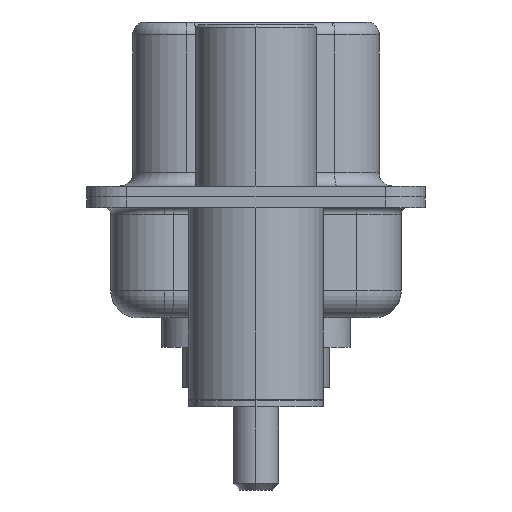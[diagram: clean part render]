
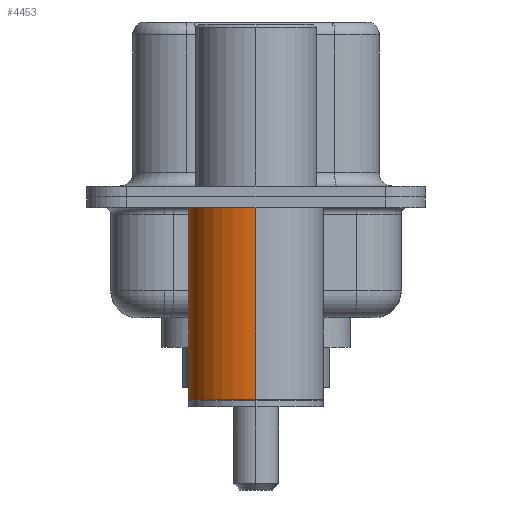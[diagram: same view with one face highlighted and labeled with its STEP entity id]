
A CAD part, left-side view. The second image highlights one B-rep face of the part: STEP entity #4453.
In plain terms, the highlighted cylindrical face has radius 2.5 mm (diameter 5 mm), a partial arc.
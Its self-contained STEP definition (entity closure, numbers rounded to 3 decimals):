
#446 = ORIENTED_EDGE ( 'NONE', *, *, #5143, .F. ) ;
#450 = CARTESIAN_POINT ( 'NONE',  ( 0., 0., -7.525 ) ) ;
#824 = VERTEX_POINT ( 'NONE', #5854 ) ;
#1178 = EDGE_LOOP ( 'NONE', ( #3720, #10890, #16262, #446 ) ) ;
#1267 = CARTESIAN_POINT ( 'NONE',  ( 0., 0., -0.4 ) ) ;
#1455 = CARTESIAN_POINT ( 'NONE',  ( -2.5, 0., 0.581 ) ) ;
#3045 = VECTOR ( 'NONE', #8073, 1000. ) ;
#3179 = DIRECTION ( 'NONE',  ( 0., 0., 1. ) ) ;
#3303 = DIRECTION ( 'NONE',  ( 1., 0., 0. ) ) ;
#3665 = VERTEX_POINT ( 'NONE', #6737 ) ;
#3720 = ORIENTED_EDGE ( 'NONE', *, *, #14409, .T. ) ;
#3956 = CARTESIAN_POINT ( 'NONE',  ( 2.5, 0., 0.581 ) ) ;
#4332 = CIRCLE ( 'NONE', #11061, 2.5 ) ;
#4346 = CARTESIAN_POINT ( 'NONE',  ( -2.5, 0., -7.525 ) ) ;
#4350 = LINE ( 'NONE', #3956, #3045 ) ;
#4453 = ADVANCED_FACE ( 'NONE', ( #7382 ), #9157, .T. ) ;
#4678 = CARTESIAN_POINT ( 'NONE',  ( 2.5, 0., -0.4 ) ) ;
#4859 = AXIS2_PLACEMENT_3D ( 'NONE', #450, #3179, #3303 ) ;
#5143 = EDGE_CURVE ( 'NONE', #3665, #5407, #4350, .T. ) ;
#5407 = VERTEX_POINT ( 'NONE', #4678 ) ;
#5854 = CARTESIAN_POINT ( 'NONE',  ( -2.5, 0., -0.4 ) ) ;
#6737 = CARTESIAN_POINT ( 'NONE',  ( 2.5, 0., -7.525 ) ) ;
#7042 = DIRECTION ( 'NONE',  ( 0., 0., 1. ) ) ;
#7382 = FACE_OUTER_BOUND ( 'NONE', #1178, .T. ) ;
#7699 = AXIS2_PLACEMENT_3D ( 'NONE', #10865, #16400, #9533 ) ;
#8073 = DIRECTION ( 'NONE',  ( 0., 0., 1. ) ) ;
#9157 = CYLINDRICAL_SURFACE ( 'NONE', #7699, 2.5 ) ;
#9533 = DIRECTION ( 'NONE',  ( 1., 0., 0. ) ) ;
#9594 = DIRECTION ( 'NONE',  ( 0., 0., 1. ) ) ;
#10018 = VECTOR ( 'NONE', #7042, 1000. ) ;
#10865 = CARTESIAN_POINT ( 'NONE',  ( 0., 0., 0.581 ) ) ;
#10890 = ORIENTED_EDGE ( 'NONE', *, *, #16973, .T. ) ;
#10971 = CIRCLE ( 'NONE', #4859, 2.5 ) ;
#10990 = DIRECTION ( 'NONE',  ( 1., 0., 0. ) ) ;
#11061 = AXIS2_PLACEMENT_3D ( 'NONE', #1267, #9594, #10990 ) ;
#11676 = EDGE_CURVE ( 'NONE', #5407, #824, #4332, .T. ) ;
#14329 = VERTEX_POINT ( 'NONE', #4346 ) ;
#14409 = EDGE_CURVE ( 'NONE', #3665, #14329, #10971, .T. ) ;
#16262 = ORIENTED_EDGE ( 'NONE', *, *, #11676, .F. ) ;
#16400 = DIRECTION ( 'NONE',  ( 0., 0., 1. ) ) ;
#16973 = EDGE_CURVE ( 'NONE', #14329, #824, #17382, .T. ) ;
#17382 = LINE ( 'NONE', #1455, #10018 ) ;
